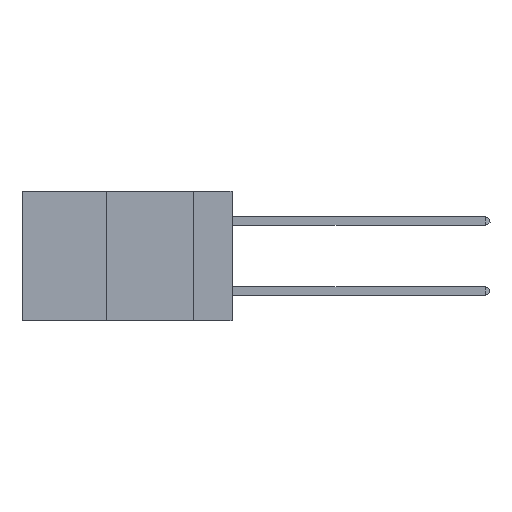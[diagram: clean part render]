
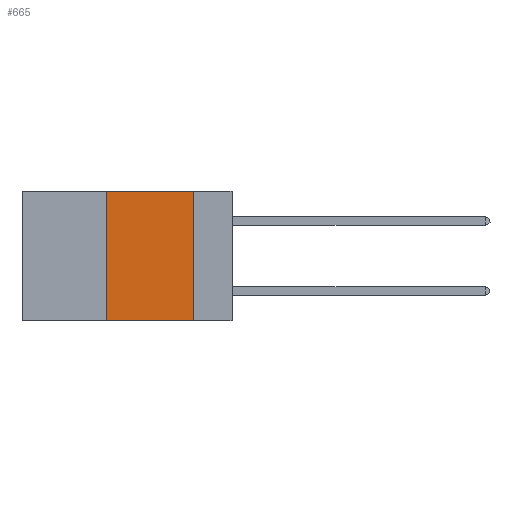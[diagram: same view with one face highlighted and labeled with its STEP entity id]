
A CAD part, left-side view. The second image highlights one B-rep face of the part: STEP entity #665.
In plain terms, the highlighted planar face has unit normal (-1, 0, 0).
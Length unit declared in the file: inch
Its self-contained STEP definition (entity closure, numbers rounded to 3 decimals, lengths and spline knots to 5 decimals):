
#665 = ADVANCED_FACE ( 'NONE', ( #2198 ), #7809, .F. ) ;
#1220 = EDGE_CURVE ( 'NONE', #1599, #15076, #13234, .T. ) ;
#1599 = VERTEX_POINT ( 'NONE', #12941 ) ;
#1746 = VECTOR ( 'NONE', #14349, 39.37008 ) ;
#1994 = DIRECTION ( 'NONE',  ( 0., 0., -1. ) ) ;
#1997 = DIRECTION ( 'NONE',  ( 0., 0., 1. ) ) ;
#2073 = VERTEX_POINT ( 'NONE', #3664 ) ;
#2198 = FACE_OUTER_BOUND ( 'NONE', #6773, .T. ) ;
#2797 = VECTOR ( 'NONE', #1994, 39.37008 ) ;
#3460 = LINE ( 'NONE', #6314, #7393 ) ;
#3664 = CARTESIAN_POINT ( 'NONE',  ( 0., 0.11, 0. ) ) ;
#4361 = VECTOR ( 'NONE', #1997, 39.37008 ) ;
#5184 = CARTESIAN_POINT ( 'NONE',  ( 0., 0.6, -0.37 ) ) ;
#6314 = CARTESIAN_POINT ( 'NONE',  ( 0., 0.6, 0. ) ) ;
#6773 = EDGE_LOOP ( 'NONE', ( #14883, #7815, #12270, #13971 ) ) ;
#7393 = VECTOR ( 'NONE', #9003, 39.37008 ) ;
#7809 = PLANE ( 'NONE',  #9756 ) ;
#7815 = ORIENTED_EDGE ( 'NONE', *, *, #11673, .F. ) ;
#8491 = VERTEX_POINT ( 'NONE', #11772 ) ;
#8766 = DIRECTION ( 'NONE',  ( 0., 0., -1. ) ) ;
#9003 = DIRECTION ( 'NONE',  ( 0., -1., 0. ) ) ;
#9756 = AXIS2_PLACEMENT_3D ( 'NONE', #12918, #12849, #8766 ) ;
#11576 = EDGE_CURVE ( 'NONE', #1599, #8491, #15052, .T. ) ;
#11673 = EDGE_CURVE ( 'NONE', #8491, #2073, #3460, .T. ) ;
#11772 = CARTESIAN_POINT ( 'NONE',  ( 0., 0.36, 0. ) ) ;
#12270 = ORIENTED_EDGE ( 'NONE', *, *, #11576, .F. ) ;
#12302 = CARTESIAN_POINT ( 'NONE',  ( 0., 0.11, 0. ) ) ;
#12849 = DIRECTION ( 'NONE',  ( 1., 0., 0. ) ) ;
#12918 = CARTESIAN_POINT ( 'NONE',  ( 0., 0.6, 0. ) ) ;
#12941 = CARTESIAN_POINT ( 'NONE',  ( 0., 0.36, -0.37 ) ) ;
#13234 = LINE ( 'NONE', #5184, #1746 ) ;
#13577 = LINE ( 'NONE', #12302, #2797 ) ;
#13645 = CARTESIAN_POINT ( 'NONE',  ( 0., 0.11, -0.37 ) ) ;
#13837 = CARTESIAN_POINT ( 'NONE',  ( 0., 0.36, 0. ) ) ;
#13971 = ORIENTED_EDGE ( 'NONE', *, *, #1220, .T. ) ;
#14349 = DIRECTION ( 'NONE',  ( 0., -1., 0. ) ) ;
#14883 = ORIENTED_EDGE ( 'NONE', *, *, #16465, .F. ) ;
#15052 = LINE ( 'NONE', #13837, #4361 ) ;
#15076 = VERTEX_POINT ( 'NONE', #13645 ) ;
#16465 = EDGE_CURVE ( 'NONE', #2073, #15076, #13577, .T. ) ;
